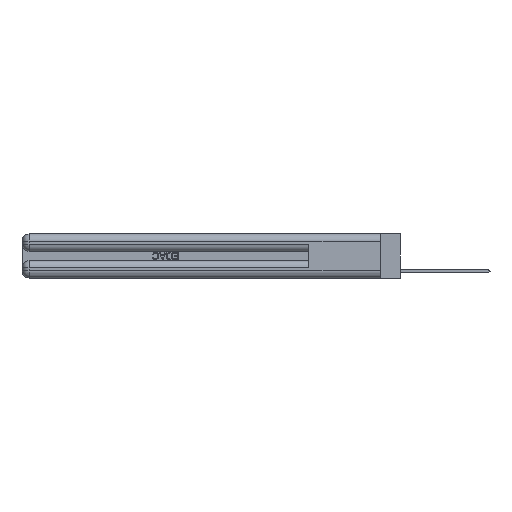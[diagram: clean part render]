
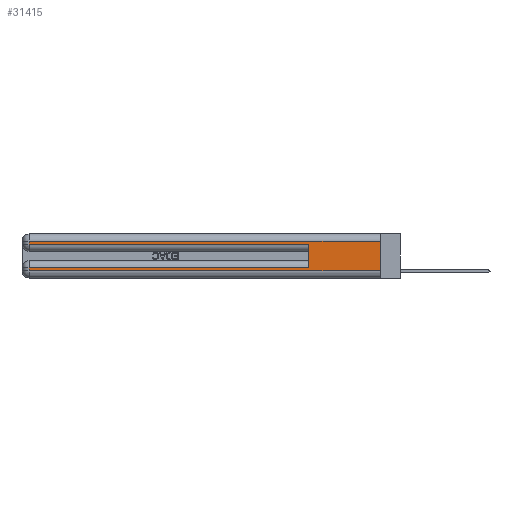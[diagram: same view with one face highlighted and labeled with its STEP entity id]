
A CAD part, left-side view. The second image highlights one B-rep face of the part: STEP entity #31415.
In plain terms, the highlighted planar face has unit normal (-1, 0, 0).
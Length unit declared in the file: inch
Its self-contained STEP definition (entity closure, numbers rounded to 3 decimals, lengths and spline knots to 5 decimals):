
#621 = CARTESIAN_POINT ( 'NONE',  ( 0., 0., 0.06 ) ) ;
#1662 = FACE_OUTER_BOUND ( 'NONE', #18683, .T. ) ;
#2067 = VECTOR ( 'NONE', #27548, 39.37008 ) ;
#2650 = EDGE_CURVE ( 'NONE', #5299, #15420, #26922, .T. ) ;
#4946 = VECTOR ( 'NONE', #29222, 39.37008 ) ;
#5248 = VERTEX_POINT ( 'NONE', #25482 ) ;
#5299 = VERTEX_POINT ( 'NONE', #11864 ) ;
#5957 = DIRECTION ( 'NONE',  ( 0., -1., 0. ) ) ;
#6990 = VECTOR ( 'NONE', #9871, 39.37008 ) ;
#7982 = PLANE ( 'NONE',  #10523 ) ;
#9305 = CARTESIAN_POINT ( 'NONE',  ( 0., 0., 0.31 ) ) ;
#9871 = DIRECTION ( 'NONE',  ( 0., 1., 0. ) ) ;
#10092 = ORIENTED_EDGE ( 'NONE', *, *, #27656, .F. ) ;
#10523 = AXIS2_PLACEMENT_3D ( 'NONE', #26514, #16127, #21413 ) ;
#11253 = VECTOR ( 'NONE', #20353, 39.37008 ) ;
#11864 = CARTESIAN_POINT ( 'NONE',  ( 0., 2.94, 0.085 ) ) ;
#12516 = LINE ( 'NONE', #22560, #2067 ) ;
#12958 = CARTESIAN_POINT ( 'NONE',  ( 0., 2.94, 0.06 ) ) ;
#14220 = LINE ( 'NONE', #22296, #33641 ) ;
#14316 = LINE ( 'NONE', #621, #27134 ) ;
#14524 = ORIENTED_EDGE ( 'NONE', *, *, #33258, .T. ) ;
#14745 = ORIENTED_EDGE ( 'NONE', *, *, #27621, .F. ) ;
#14952 = ORIENTED_EDGE ( 'NONE', *, *, #15157, .T. ) ;
#15008 = VERTEX_POINT ( 'NONE', #9305 ) ;
#15157 = EDGE_CURVE ( 'NONE', #15008, #5248, #19438, .T. ) ;
#15327 = VERTEX_POINT ( 'NONE', #22341 ) ;
#15381 = VERTEX_POINT ( 'NONE', #21158 ) ;
#15420 = VERTEX_POINT ( 'NONE', #12958 ) ;
#16127 = DIRECTION ( 'NONE',  ( 1., 0., 0. ) ) ;
#16827 = DIRECTION ( 'NONE',  ( 0., 0., -1. ) ) ;
#18683 = EDGE_LOOP ( 'NONE', ( #10092, #14952, #14524, #25862, #14745, #31847, #31877, #20569 ) ) ;
#18825 = DIRECTION ( 'NONE',  ( 0., 0., -1. ) ) ;
#19095 = LINE ( 'NONE', #21600, #4946 ) ;
#19438 = LINE ( 'NONE', #33580, #6990 ) ;
#20183 = VECTOR ( 'NONE', #18825, 39.37008 ) ;
#20241 = CARTESIAN_POINT ( 'NONE',  ( 0., 0., 0.37 ) ) ;
#20353 = DIRECTION ( 'NONE',  ( 0., 0., -1. ) ) ;
#20569 = ORIENTED_EDGE ( 'NONE', *, *, #25143, .T. ) ;
#21158 = CARTESIAN_POINT ( 'NONE',  ( 0., 0.6, 0.085 ) ) ;
#21413 = DIRECTION ( 'NONE',  ( 0., 0., -1. ) ) ;
#21600 = CARTESIAN_POINT ( 'NONE',  ( 0., 0., 0.285 ) ) ;
#21606 = LINE ( 'NONE', #20241, #11253 ) ;
#22296 = CARTESIAN_POINT ( 'NONE',  ( 0., 0., 0.085 ) ) ;
#22341 = CARTESIAN_POINT ( 'NONE',  ( 0., 0., 0.06 ) ) ;
#22560 = CARTESIAN_POINT ( 'NONE',  ( 0., 0.6, 0.145 ) ) ;
#23178 = VECTOR ( 'NONE', #16827, 39.37008 ) ;
#23247 = CARTESIAN_POINT ( 'NONE',  ( 0., 2.94, 0.285 ) ) ;
#24673 = VERTEX_POINT ( 'NONE', #23247 ) ;
#25143 = EDGE_CURVE ( 'NONE', #15420, #15327, #14316, .T. ) ;
#25482 = CARTESIAN_POINT ( 'NONE',  ( 0., 2.94, 0.31 ) ) ;
#25862 = ORIENTED_EDGE ( 'NONE', *, *, #28027, .T. ) ;
#26471 = CARTESIAN_POINT ( 'NONE',  ( 0., 0.6, 0.285 ) ) ;
#26514 = CARTESIAN_POINT ( 'NONE',  ( 0., 0., 0.37 ) ) ;
#26922 = LINE ( 'NONE', #27001, #23178 ) ;
#27001 = CARTESIAN_POINT ( 'NONE',  ( 0., 2.94, 0.37 ) ) ;
#27134 = VECTOR ( 'NONE', #5957, 39.37008 ) ;
#27548 = DIRECTION ( 'NONE',  ( 0., 0., 1. ) ) ;
#27621 = EDGE_CURVE ( 'NONE', #15381, #32160, #12516, .T. ) ;
#27622 = DIRECTION ( 'NONE',  ( 0., 1., 0. ) ) ;
#27656 = EDGE_CURVE ( 'NONE', #15008, #15327, #21606, .T. ) ;
#28027 = EDGE_CURVE ( 'NONE', #24673, #32160, #19095, .T. ) ;
#28369 = CARTESIAN_POINT ( 'NONE',  ( 0., 2.94, 0.37 ) ) ;
#29222 = DIRECTION ( 'NONE',  ( 0., -1., 0. ) ) ;
#30417 = EDGE_CURVE ( 'NONE', #15381, #5299, #14220, .T. ) ;
#31344 = LINE ( 'NONE', #28369, #20183 ) ;
#31415 = ADVANCED_FACE ( 'NONE', ( #1662 ), #7982, .F. ) ;
#31847 = ORIENTED_EDGE ( 'NONE', *, *, #30417, .T. ) ;
#31877 = ORIENTED_EDGE ( 'NONE', *, *, #2650, .T. ) ;
#32160 = VERTEX_POINT ( 'NONE', #26471 ) ;
#33258 = EDGE_CURVE ( 'NONE', #5248, #24673, #31344, .T. ) ;
#33580 = CARTESIAN_POINT ( 'NONE',  ( 0., 0., 0.31 ) ) ;
#33641 = VECTOR ( 'NONE', #27622, 39.37008 ) ;
